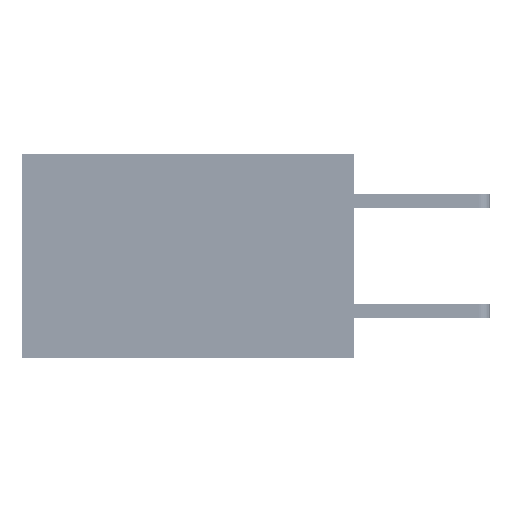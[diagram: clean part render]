
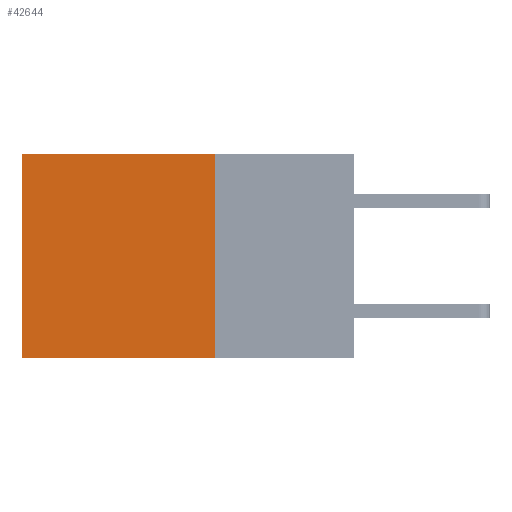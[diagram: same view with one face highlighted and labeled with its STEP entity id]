
A CAD part, left-side view. The second image highlights one B-rep face of the part: STEP entity #42644.
In plain terms, the highlighted planar face has unit normal (-1, 0, 0).
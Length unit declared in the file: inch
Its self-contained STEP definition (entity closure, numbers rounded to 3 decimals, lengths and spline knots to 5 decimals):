
#9 = VECTOR ( 'NONE', #35090, 39.37008 ) ;
#1389 = ORIENTED_EDGE ( 'NONE', *, *, #16222, .T. ) ;
#6610 = ORIENTED_EDGE ( 'NONE', *, *, #11176, .T. ) ;
#7251 = DIRECTION ( 'NONE',  ( 1., 0., 0. ) ) ;
#8531 = CARTESIAN_POINT ( 'NONE',  ( 0.2875, 0.6, -0.37 ) ) ;
#8723 = CARTESIAN_POINT ( 'NONE',  ( 0.2875, 0.25, 0. ) ) ;
#11176 = EDGE_CURVE ( 'NONE', #20804, #44993, #12720, .T. ) ;
#12720 = LINE ( 'NONE', #15513, #34451 ) ;
#13866 = EDGE_LOOP ( 'NONE', ( #6610, #22293, #20770, #1389 ) ) ;
#15513 = CARTESIAN_POINT ( 'NONE',  ( 0.2875, 0.6, 0. ) ) ;
#16222 = EDGE_CURVE ( 'NONE', #37041, #20804, #20952, .T. ) ;
#16594 = CARTESIAN_POINT ( 'NONE',  ( 0.2875, 0.6, 0. ) ) ;
#17215 = DIRECTION ( 'NONE',  ( 0., 0., -1. ) ) ;
#18121 = CARTESIAN_POINT ( 'NONE',  ( 0.2875, 0.25, 0. ) ) ;
#18781 = EDGE_CURVE ( 'NONE', #37041, #30187, #39301, .T. ) ;
#20770 = ORIENTED_EDGE ( 'NONE', *, *, #18781, .F. ) ;
#20804 = VERTEX_POINT ( 'NONE', #16594 ) ;
#20952 = LINE ( 'NONE', #31152, #9 ) ;
#21698 = CARTESIAN_POINT ( 'NONE',  ( 0.2875, 0.25, 0. ) ) ;
#22293 = ORIENTED_EDGE ( 'NONE', *, *, #26766, .F. ) ;
#24396 = CARTESIAN_POINT ( 'NONE',  ( 0.2875, 0.25, -0.37 ) ) ;
#25874 = CARTESIAN_POINT ( 'NONE',  ( 0.2875, 0.25, -0.37 ) ) ;
#26766 = EDGE_CURVE ( 'NONE', #30187, #44993, #42009, .T. ) ;
#28538 = FACE_OUTER_BOUND ( 'NONE', #13866, .T. ) ;
#29086 = VECTOR ( 'NONE', #35603, 39.37008 ) ;
#30187 = VERTEX_POINT ( 'NONE', #25874 ) ;
#31152 = CARTESIAN_POINT ( 'NONE',  ( 0.2875, 0.25, 0. ) ) ;
#34185 = AXIS2_PLACEMENT_3D ( 'NONE', #18121, #7251, #17215 ) ;
#34451 = VECTOR ( 'NONE', #40514, 39.37008 ) ;
#34804 = PLANE ( 'NONE',  #34185 ) ;
#35090 = DIRECTION ( 'NONE',  ( 0., 1., 0. ) ) ;
#35603 = DIRECTION ( 'NONE',  ( 0., 0., -1. ) ) ;
#37041 = VERTEX_POINT ( 'NONE', #8723 ) ;
#37632 = DIRECTION ( 'NONE',  ( 0., 1., 0. ) ) ;
#39301 = LINE ( 'NONE', #21698, #29086 ) ;
#40514 = DIRECTION ( 'NONE',  ( 0., 0., -1. ) ) ;
#41850 = VECTOR ( 'NONE', #37632, 39.37008 ) ;
#42009 = LINE ( 'NONE', #24396, #41850 ) ;
#42644 = ADVANCED_FACE ( 'NONE', ( #28538 ), #34804, .F. ) ;
#44993 = VERTEX_POINT ( 'NONE', #8531 ) ;
